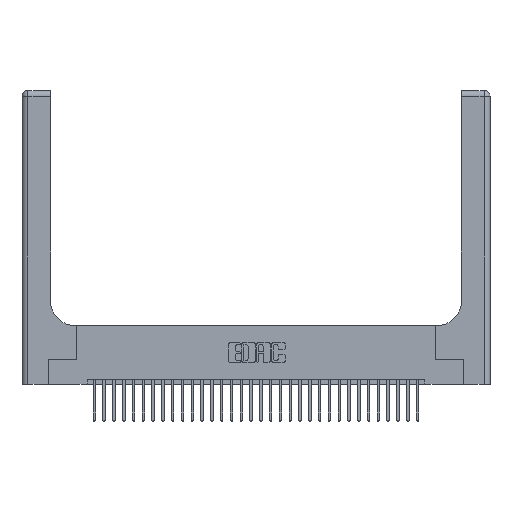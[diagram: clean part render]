
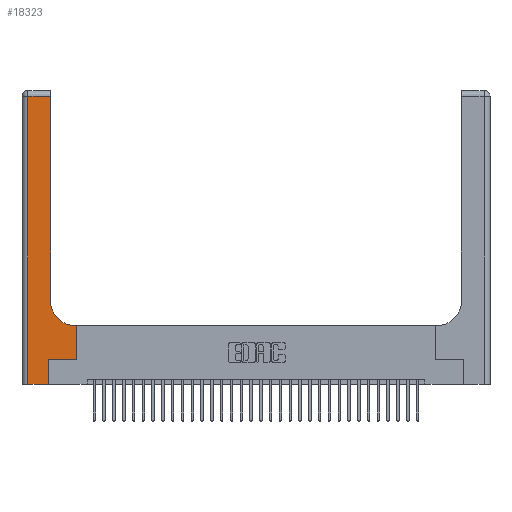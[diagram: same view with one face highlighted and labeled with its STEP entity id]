
A CAD part, top view. The second image highlights one B-rep face of the part: STEP entity #18323.
In plain terms, the highlighted planar face has unit normal (0, 0, 1).
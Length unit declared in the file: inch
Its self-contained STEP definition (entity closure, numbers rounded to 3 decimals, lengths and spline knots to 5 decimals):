
#344 = LINE ( 'NONE', #27621, #26698 ) ;
#664 = CARTESIAN_POINT ( 'NONE',  ( 0., 3., 0.37 ) ) ;
#876 = CARTESIAN_POINT ( 'NONE',  ( 0.269, 0., 0.37 ) ) ;
#1047 = CARTESIAN_POINT ( 'NONE',  ( 0.269, 0.25, 0.37 ) ) ;
#1268 = DIRECTION ( 'NONE',  ( -1., 0., 0. ) ) ;
#1347 = LINE ( 'NONE', #13063, #31627 ) ;
#1407 = VECTOR ( 'NONE', #28008, 39.37008 ) ;
#1510 = LINE ( 'NONE', #19637, #7470 ) ;
#2446 = ORIENTED_EDGE ( 'NONE', *, *, #24538, .T. ) ;
#2549 = CARTESIAN_POINT ( 'NONE',  ( 0.06, 3., 0.37 ) ) ;
#3744 = DIRECTION ( 'NONE',  ( 0., 1., 0. ) ) ;
#4390 = LINE ( 'NONE', #18919, #11959 ) ;
#6332 = DIRECTION ( 'NONE',  ( 0., 0., -1. ) ) ;
#7168 = VERTEX_POINT ( 'NONE', #9124 ) ;
#7470 = VECTOR ( 'NONE', #27472, 39.37008 ) ;
#7562 = CARTESIAN_POINT ( 'NONE',  ( 0.06, 0., 0.37 ) ) ;
#7686 = EDGE_LOOP ( 'NONE', ( #25557, #8465, #23474, #27183, #26648, #15779, #25480, #28838, #2446 ) ) ;
#7776 = EDGE_CURVE ( 'NONE', #16788, #7168, #22994, .T. ) ;
#8207 = VERTEX_POINT ( 'NONE', #15404 ) ;
#8465 = ORIENTED_EDGE ( 'NONE', *, *, #25972, .T. ) ;
#8594 = DIRECTION ( 'NONE',  ( 0., 1., 0. ) ) ;
#8827 = CARTESIAN_POINT ( 'NONE',  ( 0.2915, 0.6, 0.37 ) ) ;
#8910 = CARTESIAN_POINT ( 'NONE',  ( 0.5585, 0.25, 0.37 ) ) ;
#9124 = CARTESIAN_POINT ( 'NONE',  ( 0.5585, 0.6, 0.37 ) ) ;
#9326 = CARTESIAN_POINT ( 'NONE',  ( 0.2915, 2.94, 0.37 ) ) ;
#10558 = DIRECTION ( 'NONE',  ( 0., 0., -1. ) ) ;
#10897 = LINE ( 'NONE', #13873, #28444 ) ;
#11571 = DIRECTION ( 'NONE',  ( 1., 0., 0. ) ) ;
#11937 = VECTOR ( 'NONE', #8594, 39.37008 ) ;
#11959 = VECTOR ( 'NONE', #29294, 39.37008 ) ;
#12395 = DIRECTION ( 'NONE',  ( 1., 0., 0. ) ) ;
#13063 = CARTESIAN_POINT ( 'NONE',  ( 0.269, 0., 0.37 ) ) ;
#13075 = VERTEX_POINT ( 'NONE', #21363 ) ;
#13873 = CARTESIAN_POINT ( 'NONE',  ( 0.2915, 3., 0.37 ) ) ;
#14285 = CARTESIAN_POINT ( 'NONE',  ( 0.5415, 0.6, 0.37 ) ) ;
#14368 = EDGE_CURVE ( 'NONE', #8207, #22416, #10897, .T. ) ;
#14836 = EDGE_CURVE ( 'NONE', #23948, #26841, #1347, .T. ) ;
#15249 = VERTEX_POINT ( 'NONE', #14285 ) ;
#15385 = EDGE_CURVE ( 'NONE', #26841, #16788, #344, .T. ) ;
#15404 = CARTESIAN_POINT ( 'NONE',  ( 0.2915, 0.85, 0.37 ) ) ;
#15779 = ORIENTED_EDGE ( 'NONE', *, *, #15385, .T. ) ;
#16788 = VERTEX_POINT ( 'NONE', #8910 ) ;
#18323 = ADVANCED_FACE ( 'NONE', ( #28086 ), #25856, .F. ) ;
#18919 = CARTESIAN_POINT ( 'NONE',  ( 0., 2.94, 0.37 ) ) ;
#19637 = CARTESIAN_POINT ( 'NONE',  ( 0., 0., 0.37 ) ) ;
#19771 = AXIS2_PLACEMENT_3D ( 'NONE', #31245, #6332, #11571 ) ;
#21203 = CARTESIAN_POINT ( 'NONE',  ( 0.5585, 0.25, 0.37 ) ) ;
#21363 = CARTESIAN_POINT ( 'NONE',  ( 0.06, 2.94, 0.37 ) ) ;
#22416 = VERTEX_POINT ( 'NONE', #9326 ) ;
#22437 = LINE ( 'NONE', #8827, #30035 ) ;
#22555 = EDGE_CURVE ( 'NONE', #13075, #27727, #29301, .T. ) ;
#22917 = DIRECTION ( 'NONE',  ( 0., 1., 0. ) ) ;
#22994 = LINE ( 'NONE', #21203, #11937 ) ;
#23474 = ORIENTED_EDGE ( 'NONE', *, *, #22555, .T. ) ;
#23948 = VERTEX_POINT ( 'NONE', #876 ) ;
#24538 = EDGE_CURVE ( 'NONE', #15249, #8207, #27170, .T. ) ;
#25480 = ORIENTED_EDGE ( 'NONE', *, *, #7776, .T. ) ;
#25557 = ORIENTED_EDGE ( 'NONE', *, *, #14368, .T. ) ;
#25856 = PLANE ( 'NONE',  #28378 ) ;
#25972 = EDGE_CURVE ( 'NONE', #22416, #13075, #4390, .T. ) ;
#26648 = ORIENTED_EDGE ( 'NONE', *, *, #14836, .T. ) ;
#26698 = VECTOR ( 'NONE', #12395, 39.37008 ) ;
#26841 = VERTEX_POINT ( 'NONE', #1047 ) ;
#27170 = CIRCLE ( 'NONE', #19771, 0.25 ) ;
#27183 = ORIENTED_EDGE ( 'NONE', *, *, #30191, .T. ) ;
#27472 = DIRECTION ( 'NONE',  ( 1., 0., 0. ) ) ;
#27621 = CARTESIAN_POINT ( 'NONE',  ( 0.269, 0.25, 0.37 ) ) ;
#27727 = VERTEX_POINT ( 'NONE', #7562 ) ;
#28008 = DIRECTION ( 'NONE',  ( 0., -1., 0. ) ) ;
#28086 = FACE_OUTER_BOUND ( 'NONE', #7686, .T. ) ;
#28178 = DIRECTION ( 'NONE',  ( -1., 0., 0. ) ) ;
#28378 = AXIS2_PLACEMENT_3D ( 'NONE', #664, #10558, #28178 ) ;
#28444 = VECTOR ( 'NONE', #3744, 39.37008 ) ;
#28838 = ORIENTED_EDGE ( 'NONE', *, *, #32140, .T. ) ;
#29294 = DIRECTION ( 'NONE',  ( -1., 0., 0. ) ) ;
#29301 = LINE ( 'NONE', #2549, #1407 ) ;
#30035 = VECTOR ( 'NONE', #1268, 39.37008 ) ;
#30191 = EDGE_CURVE ( 'NONE', #27727, #23948, #1510, .T. ) ;
#31245 = CARTESIAN_POINT ( 'NONE',  ( 0.5415, 0.85, 0.37 ) ) ;
#31627 = VECTOR ( 'NONE', #22917, 39.37008 ) ;
#32140 = EDGE_CURVE ( 'NONE', #7168, #15249, #22437, .T. ) ;
